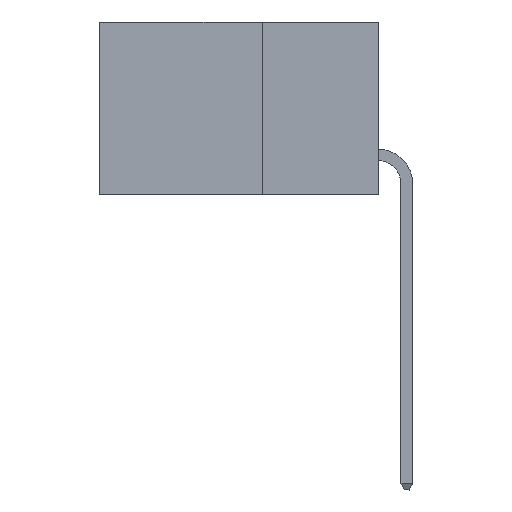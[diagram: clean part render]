
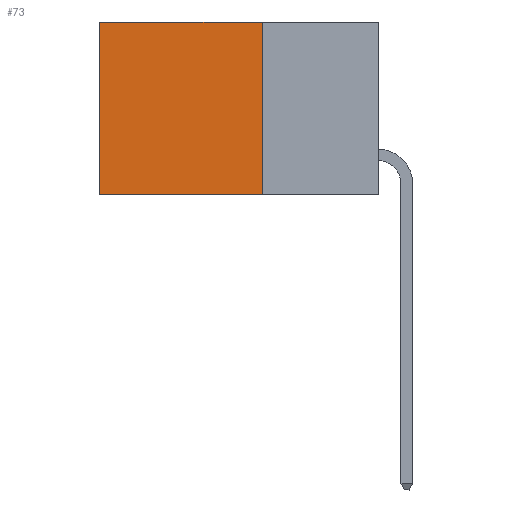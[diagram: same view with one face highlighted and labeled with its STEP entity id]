
A CAD part, left-side view. The second image highlights one B-rep face of the part: STEP entity #73.
In plain terms, the highlighted planar face has unit normal (-1, 0, 0).
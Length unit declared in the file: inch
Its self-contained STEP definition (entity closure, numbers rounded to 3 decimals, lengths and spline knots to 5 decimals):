
#73 = ADVANCED_FACE ( 'NONE', ( #15107 ), #15198, .F. ) ;
#266 = ORIENTED_EDGE ( 'NONE', *, *, #8501, .T. ) ;
#460 = CARTESIAN_POINT ( 'NONE',  ( 0.298, 0.25, 0. ) ) ;
#884 = CARTESIAN_POINT ( 'NONE',  ( 0.298, 0.25, 0. ) ) ;
#1118 = AXIS2_PLACEMENT_3D ( 'NONE', #4879, #4992, #3618 ) ;
#1430 = EDGE_CURVE ( 'NONE', #11889, #13498, #2222, .T. ) ;
#2054 = LINE ( 'NONE', #7015, #8476 ) ;
#2222 = LINE ( 'NONE', #16571, #7023 ) ;
#2769 = ORIENTED_EDGE ( 'NONE', *, *, #1430, .T. ) ;
#3025 = DIRECTION ( 'NONE',  ( 0., 0., -1. ) ) ;
#3618 = DIRECTION ( 'NONE',  ( 0., 0., -1. ) ) ;
#3721 = EDGE_LOOP ( 'NONE', ( #2769, #14230, #6520, #266 ) ) ;
#4879 = CARTESIAN_POINT ( 'NONE',  ( 0.298, 0.25, 0. ) ) ;
#4992 = DIRECTION ( 'NONE',  ( 1., 0., 0. ) ) ;
#5562 = LINE ( 'NONE', #460, #6766 ) ;
#6520 = ORIENTED_EDGE ( 'NONE', *, *, #14958, .F. ) ;
#6766 = VECTOR ( 'NONE', #3025, 39.37008 ) ;
#7015 = CARTESIAN_POINT ( 'NONE',  ( 0.298, 0.25, -0.37 ) ) ;
#7023 = VECTOR ( 'NONE', #15276, 39.37008 ) ;
#7473 = LINE ( 'NONE', #10941, #13495 ) ;
#7924 = DIRECTION ( 'NONE',  ( 0., 1., 0. ) ) ;
#8180 = DIRECTION ( 'NONE',  ( 0., 1., 0. ) ) ;
#8476 = VECTOR ( 'NONE', #7924, 39.37008 ) ;
#8501 = EDGE_CURVE ( 'NONE', #8548, #11889, #7473, .T. ) ;
#8548 = VERTEX_POINT ( 'NONE', #884 ) ;
#8923 = EDGE_CURVE ( 'NONE', #15748, #13498, #2054, .T. ) ;
#10941 = CARTESIAN_POINT ( 'NONE',  ( 0.298, 0.25, 0. ) ) ;
#11889 = VERTEX_POINT ( 'NONE', #12926 ) ;
#12776 = CARTESIAN_POINT ( 'NONE',  ( 0.298, 0.6, -0.37 ) ) ;
#12926 = CARTESIAN_POINT ( 'NONE',  ( 0.298, 0.6, 0. ) ) ;
#13495 = VECTOR ( 'NONE', #8180, 39.37008 ) ;
#13498 = VERTEX_POINT ( 'NONE', #12776 ) ;
#14230 = ORIENTED_EDGE ( 'NONE', *, *, #8923, .F. ) ;
#14375 = CARTESIAN_POINT ( 'NONE',  ( 0.298, 0.25, -0.37 ) ) ;
#14958 = EDGE_CURVE ( 'NONE', #8548, #15748, #5562, .T. ) ;
#15107 = FACE_OUTER_BOUND ( 'NONE', #3721, .T. ) ;
#15198 = PLANE ( 'NONE',  #1118 ) ;
#15276 = DIRECTION ( 'NONE',  ( 0., 0., -1. ) ) ;
#15748 = VERTEX_POINT ( 'NONE', #14375 ) ;
#16571 = CARTESIAN_POINT ( 'NONE',  ( 0.298, 0.6, 0. ) ) ;
